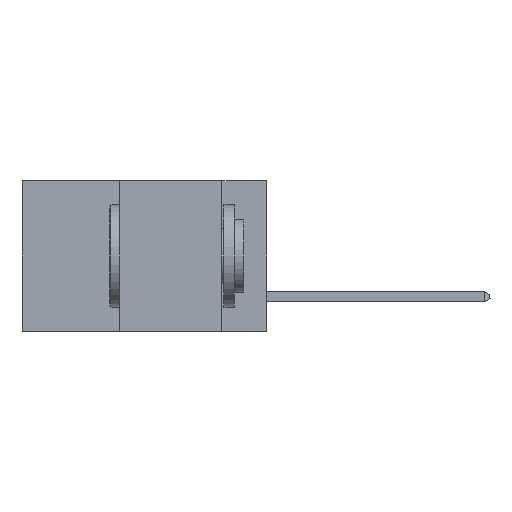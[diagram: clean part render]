
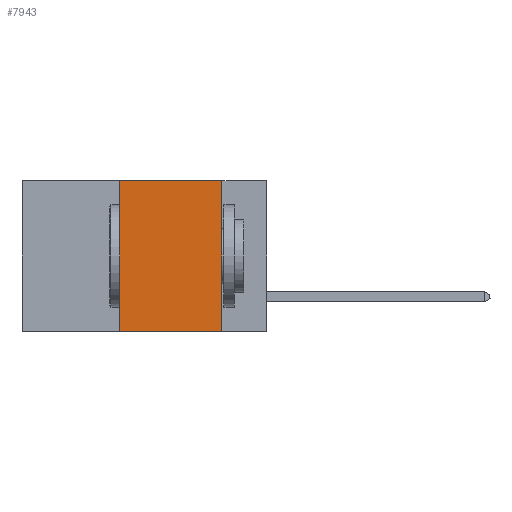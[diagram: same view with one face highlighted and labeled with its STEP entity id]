
A CAD part, left-side view. The second image highlights one B-rep face of the part: STEP entity #7943.
In plain terms, the highlighted planar face has unit normal (-1, 0, 0).
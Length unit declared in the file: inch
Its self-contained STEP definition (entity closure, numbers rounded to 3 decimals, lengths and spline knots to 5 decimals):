
#446 = CARTESIAN_POINT ( 'NONE',  ( 0., 0.6, 0. ) ) ;
#2333 = DIRECTION ( 'NONE',  ( 0., -1., 0. ) ) ;
#3252 = EDGE_CURVE ( 'NONE', #14424, #7448, #10661, .T. ) ;
#3310 = CARTESIAN_POINT ( 'NONE',  ( 0., 0.11, 0. ) ) ;
#3800 = EDGE_CURVE ( 'NONE', #12381, #14424, #14057, .T. ) ;
#3832 = CARTESIAN_POINT ( 'NONE',  ( 0., 0.11, 0. ) ) ;
#4130 = EDGE_CURVE ( 'NONE', #15283, #7448, #15520, .T. ) ;
#5670 = CARTESIAN_POINT ( 'NONE',  ( 0., 0.36, -0.37 ) ) ;
#5756 = LINE ( 'NONE', #6655, #15196 ) ;
#5952 = DIRECTION ( 'NONE',  ( 0., 0., -1. ) ) ;
#6655 = CARTESIAN_POINT ( 'NONE',  ( 0., 0.36, 0. ) ) ;
#6944 = EDGE_CURVE ( 'NONE', #15283, #12381, #5756, .T. ) ;
#7079 = VECTOR ( 'NONE', #5952, 39.37008 ) ;
#7448 = VERTEX_POINT ( 'NONE', #8994 ) ;
#7494 = DIRECTION ( 'NONE',  ( 0., 0., 1. ) ) ;
#7573 = DIRECTION ( 'NONE',  ( 1., 0., 0. ) ) ;
#7743 = PLANE ( 'NONE',  #9294 ) ;
#7943 = ADVANCED_FACE ( 'NONE', ( #12923 ), #7743, .F. ) ;
#8994 = CARTESIAN_POINT ( 'NONE',  ( 0., 0.11, -0.37 ) ) ;
#9294 = AXIS2_PLACEMENT_3D ( 'NONE', #446, #7573, #12464 ) ;
#9680 = EDGE_LOOP ( 'NONE', ( #14442, #10026, #11259, #14229 ) ) ;
#10026 = ORIENTED_EDGE ( 'NONE', *, *, #3800, .F. ) ;
#10591 = DIRECTION ( 'NONE',  ( 0., -1., 0. ) ) ;
#10610 = CARTESIAN_POINT ( 'NONE',  ( 0., 0.36, 0. ) ) ;
#10661 = LINE ( 'NONE', #3310, #7079 ) ;
#10798 = CARTESIAN_POINT ( 'NONE',  ( 0., 0.6, 0. ) ) ;
#11014 = VECTOR ( 'NONE', #2333, 39.37008 ) ;
#11259 = ORIENTED_EDGE ( 'NONE', *, *, #6944, .F. ) ;
#12381 = VERTEX_POINT ( 'NONE', #10610 ) ;
#12464 = DIRECTION ( 'NONE',  ( 0., 0., -1. ) ) ;
#12918 = VECTOR ( 'NONE', #10591, 39.37008 ) ;
#12923 = FACE_OUTER_BOUND ( 'NONE', #9680, .T. ) ;
#13005 = CARTESIAN_POINT ( 'NONE',  ( 0., 0.6, -0.37 ) ) ;
#14057 = LINE ( 'NONE', #10798, #11014 ) ;
#14229 = ORIENTED_EDGE ( 'NONE', *, *, #4130, .T. ) ;
#14424 = VERTEX_POINT ( 'NONE', #3832 ) ;
#14442 = ORIENTED_EDGE ( 'NONE', *, *, #3252, .F. ) ;
#15196 = VECTOR ( 'NONE', #7494, 39.37008 ) ;
#15283 = VERTEX_POINT ( 'NONE', #5670 ) ;
#15520 = LINE ( 'NONE', #13005, #12918 ) ;
